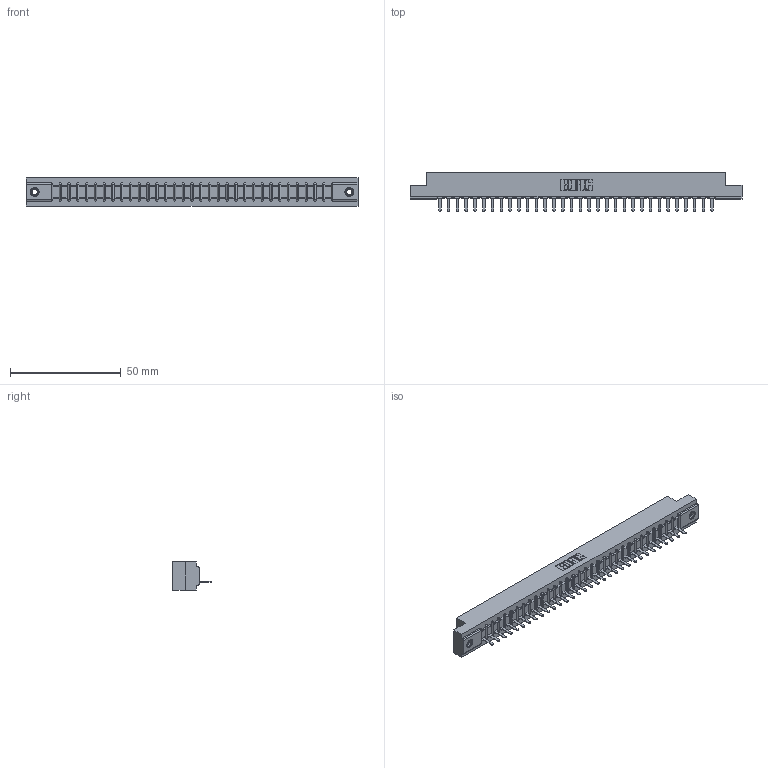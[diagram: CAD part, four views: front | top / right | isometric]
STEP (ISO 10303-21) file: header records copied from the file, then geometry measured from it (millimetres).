
FILE_DESCRIPTION (( 'STEP AP203' ), '1' );
FILE_NAME ('307-032-521-107.STEP', '2019-09-05T05:16:18', ( '' ), ( '' ), 'SwSTEP 2.0', 'SolidWorks 2016', '' );
FILE_SCHEMA (( 'CONFIG_CONTROL_DESIGN' ));
Length unit declared in the file: inch
Products named in the file (4): 307-032-521-107; 345-250-001_345-250-005-103; 307 Part_.156 Dia Mounting Holes; 307-290-002_521
Assembly tree (35 placements, depth 2):
  307-032-521-107
    307 Part_.156 Dia Mounting Holes
    307-290-002_521  x32
    345-250-001_345-250-005-103  x2
Bounding box: 149.81 x 17.42 x 12.7 mm (x, y, z)
Volume: 15945.3 mm3; surface area: 19867.9 mm2
Topology: 35 solids, 35 shells, 2579 faces, 7883 edges, 5158 vertices
Faces by surface type: plane 1542, cylinder 955, sphere 66, cone 12, torus 4
Entity records: 30569 total; most frequent: CARTESIAN_POINT 5135, ORIENTED_EDGE 5118, DIRECTION 5003, EDGE_CURVE 2559, VECTOR 1955, LINE 1955, VERTEX_POINT 1656, AXIS2_PLACEMENT_3D 1524
